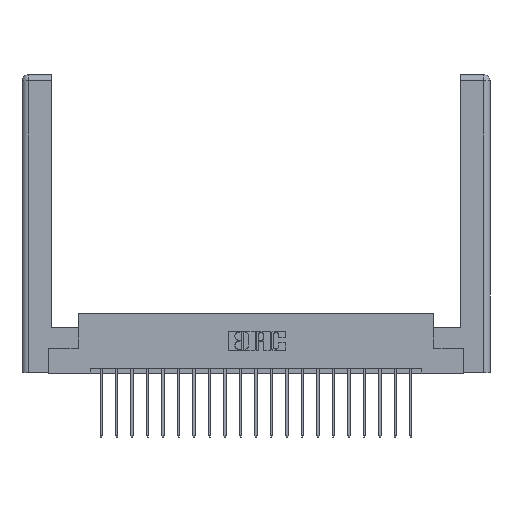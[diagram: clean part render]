
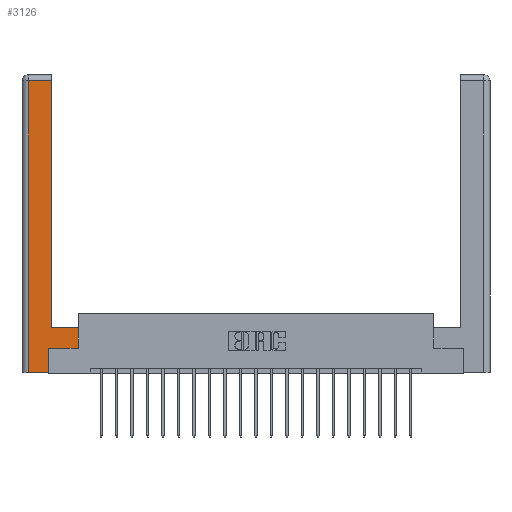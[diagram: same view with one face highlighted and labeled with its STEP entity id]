
A CAD part, top view. The second image highlights one B-rep face of the part: STEP entity #3126.
In plain terms, the highlighted planar face has unit normal (0, 0, 1).
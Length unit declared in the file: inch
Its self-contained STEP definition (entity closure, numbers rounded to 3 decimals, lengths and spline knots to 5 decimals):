
#45 = CARTESIAN_POINT ( 'NONE',  ( 0.565, 0.45, 0. ) ) ;
#74 = VECTOR ( 'NONE', #2199, 39.37008 ) ;
#215 = VECTOR ( 'NONE', #10340, 39.37008 ) ;
#350 = CARTESIAN_POINT ( 'NONE',  ( 0.265, 0.245, 0. ) ) ;
#422 = CARTESIAN_POINT ( 'NONE',  ( 0.295, 0.45, 0. ) ) ;
#579 = CARTESIAN_POINT ( 'NONE',  ( 0.295, 2.94, 0. ) ) ;
#648 = EDGE_CURVE ( 'NONE', #1368, #11447, #3819, .T. ) ;
#1368 = VERTEX_POINT ( 'NONE', #579 ) ;
#1659 = LINE ( 'NONE', #16667, #18937 ) ;
#1809 = VERTEX_POINT ( 'NONE', #18634 ) ;
#2157 = ORIENTED_EDGE ( 'NONE', *, *, #8101, .T. ) ;
#2178 = CARTESIAN_POINT ( 'NONE',  ( 0.565, 0.245, 0. ) ) ;
#2199 = DIRECTION ( 'NONE',  ( 0., 1., 0. ) ) ;
#2427 = ORIENTED_EDGE ( 'NONE', *, *, #13102, .T. ) ;
#3094 = ORIENTED_EDGE ( 'NONE', *, *, #9292, .T. ) ;
#3126 = ADVANCED_FACE ( 'NONE', ( #16104 ), #13940, .F. ) ;
#3516 = EDGE_CURVE ( 'NONE', #14128, #1368, #11675, .T. ) ;
#3815 = VECTOR ( 'NONE', #21007, 39.37008 ) ;
#3819 = LINE ( 'NONE', #14968, #18222 ) ;
#3869 = ORIENTED_EDGE ( 'NONE', *, *, #648, .T. ) ;
#4350 = LINE ( 'NONE', #15696, #18778 ) ;
#4548 = CARTESIAN_POINT ( 'NONE',  ( 0.265, 0., 0. ) ) ;
#4743 = DIRECTION ( 'NONE',  ( -1., 0., 0. ) ) ;
#5209 = ORIENTED_EDGE ( 'NONE', *, *, #16679, .T. ) ;
#5283 = CARTESIAN_POINT ( 'NONE',  ( 0.0615, 2.94, 0. ) ) ;
#5516 = DIRECTION ( 'NONE',  ( 1., 0., 0. ) ) ;
#5522 = DIRECTION ( 'NONE',  ( 1., 0., 0. ) ) ;
#5747 = CARTESIAN_POINT ( 'NONE',  ( 0.295, 0.45, 0. ) ) ;
#6617 = DIRECTION ( 'NONE',  ( -1., 0., 0. ) ) ;
#6939 = DIRECTION ( 'NONE',  ( 0., 1., 0. ) ) ;
#6978 = DIRECTION ( 'NONE',  ( 0., -1., 0. ) ) ;
#7198 = VECTOR ( 'NONE', #5522, 39.37008 ) ;
#7616 = CARTESIAN_POINT ( 'NONE',  ( 0.295, 3., 0. ) ) ;
#8019 = VERTEX_POINT ( 'NONE', #12155 ) ;
#8060 = CARTESIAN_POINT ( 'NONE',  ( 0.565, 0.245, 0. ) ) ;
#8101 = EDGE_CURVE ( 'NONE', #8019, #14128, #18502, .T. ) ;
#9292 = EDGE_CURVE ( 'NONE', #16079, #9468, #16643, .T. ) ;
#9453 = LINE ( 'NONE', #45, #74 ) ;
#9468 = VERTEX_POINT ( 'NONE', #8060 ) ;
#9776 = EDGE_LOOP ( 'NONE', ( #19217, #3869, #2427, #5209, #14267, #3094, #15856, #2157 ) ) ;
#10340 = DIRECTION ( 'NONE',  ( -1., 0., 0. ) ) ;
#10969 = CARTESIAN_POINT ( 'NONE',  ( 0.265, 0.245, 0. ) ) ;
#11447 = VERTEX_POINT ( 'NONE', #5283 ) ;
#11675 = LINE ( 'NONE', #7616, #3815 ) ;
#12155 = CARTESIAN_POINT ( 'NONE',  ( 0.565, 0.45, 0. ) ) ;
#13102 = EDGE_CURVE ( 'NONE', #11447, #1809, #1659, .T. ) ;
#13442 = VERTEX_POINT ( 'NONE', #4548 ) ;
#13940 = PLANE ( 'NONE',  #14482 ) ;
#14128 = VERTEX_POINT ( 'NONE', #5747 ) ;
#14267 = ORIENTED_EDGE ( 'NONE', *, *, #14901, .T. ) ;
#14482 = AXIS2_PLACEMENT_3D ( 'NONE', #19858, #19699, #4743 ) ;
#14901 = EDGE_CURVE ( 'NONE', #13442, #16079, #17270, .T. ) ;
#14968 = CARTESIAN_POINT ( 'NONE',  ( 0.0615, 2.94, 0. ) ) ;
#15696 = CARTESIAN_POINT ( 'NONE',  ( 0.265, 0., 0. ) ) ;
#15856 = ORIENTED_EDGE ( 'NONE', *, *, #20229, .T. ) ;
#16079 = VERTEX_POINT ( 'NONE', #10969 ) ;
#16104 = FACE_OUTER_BOUND ( 'NONE', #9776, .T. ) ;
#16643 = LINE ( 'NONE', #2178, #7198 ) ;
#16667 = CARTESIAN_POINT ( 'NONE',  ( 0.0615, 0., 0. ) ) ;
#16679 = EDGE_CURVE ( 'NONE', #1809, #13442, #4350, .T. ) ;
#17270 = LINE ( 'NONE', #350, #19915 ) ;
#18222 = VECTOR ( 'NONE', #6617, 39.37008 ) ;
#18502 = LINE ( 'NONE', #422, #215 ) ;
#18634 = CARTESIAN_POINT ( 'NONE',  ( 0.0615, 0., 0. ) ) ;
#18778 = VECTOR ( 'NONE', #5516, 39.37008 ) ;
#18937 = VECTOR ( 'NONE', #6978, 39.37008 ) ;
#19217 = ORIENTED_EDGE ( 'NONE', *, *, #3516, .T. ) ;
#19699 = DIRECTION ( 'NONE',  ( 0., 0., -1. ) ) ;
#19858 = CARTESIAN_POINT ( 'NONE',  ( 0., 0., 0. ) ) ;
#19915 = VECTOR ( 'NONE', #6939, 39.37008 ) ;
#20229 = EDGE_CURVE ( 'NONE', #9468, #8019, #9453, .T. ) ;
#21007 = DIRECTION ( 'NONE',  ( 0., 1., 0. ) ) ;
